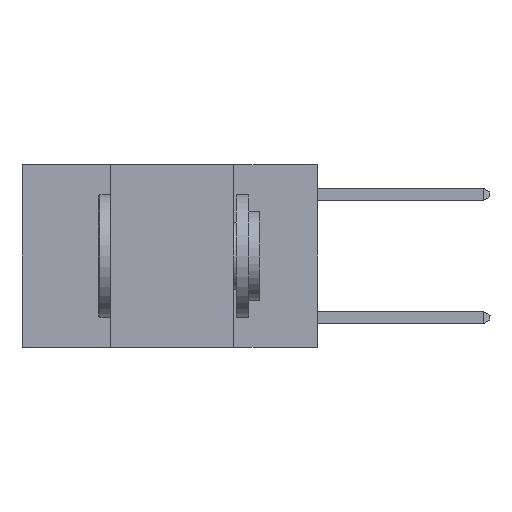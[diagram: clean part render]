
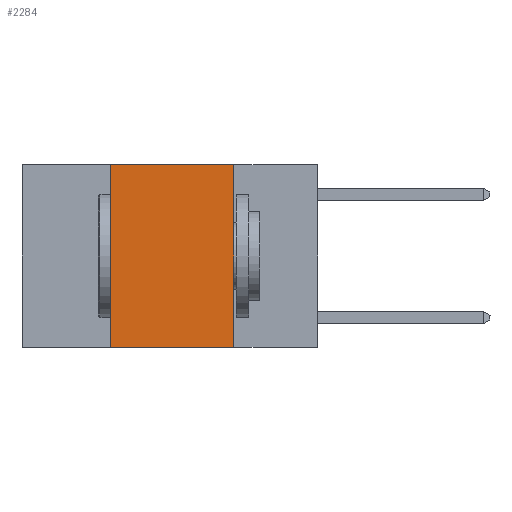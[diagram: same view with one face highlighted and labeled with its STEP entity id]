
A CAD part, left-side view. The second image highlights one B-rep face of the part: STEP entity #2284.
In plain terms, the highlighted planar face has unit normal (-1, 0, 0).
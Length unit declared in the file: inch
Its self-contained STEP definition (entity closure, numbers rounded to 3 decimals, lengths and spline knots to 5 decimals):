
#286 = VERTEX_POINT ( 'NONE', #10735 ) ;
#555 = DIRECTION ( 'NONE',  ( 0., -1., 0. ) ) ;
#801 = CARTESIAN_POINT ( 'NONE',  ( 0., 0.42, 0. ) ) ;
#992 = CARTESIAN_POINT ( 'NONE',  ( 0., 0.17, -0.37 ) ) ;
#1874 = CARTESIAN_POINT ( 'NONE',  ( 0., 0.6, -0.37 ) ) ;
#1924 = VECTOR ( 'NONE', #555, 39.37008 ) ;
#2204 = VERTEX_POINT ( 'NONE', #10578 ) ;
#2284 = ADVANCED_FACE ( 'NONE', ( #10829 ), #9091, .F. ) ;
#3092 = ORIENTED_EDGE ( 'NONE', *, *, #7456, .F. ) ;
#4289 = LINE ( 'NONE', #1874, #8643 ) ;
#4539 = LINE ( 'NONE', #801, #10482 ) ;
#4561 = DIRECTION ( 'NONE',  ( 0., -1., 0. ) ) ;
#4571 = LINE ( 'NONE', #10651, #1924 ) ;
#4818 = CARTESIAN_POINT ( 'NONE',  ( 0., 0.17, 0. ) ) ;
#5016 = AXIS2_PLACEMENT_3D ( 'NONE', #9240, #9254, #7858 ) ;
#6104 = EDGE_CURVE ( 'NONE', #9518, #2204, #4571, .T. ) ;
#6922 = EDGE_CURVE ( 'NONE', #286, #7641, #4289, .T. ) ;
#6931 = DIRECTION ( 'NONE',  ( 0., 0., 1. ) ) ;
#7133 = VECTOR ( 'NONE', #10443, 39.37008 ) ;
#7335 = ORIENTED_EDGE ( 'NONE', *, *, #7977, .F. ) ;
#7456 = EDGE_CURVE ( 'NONE', #286, #9518, #4539, .T. ) ;
#7583 = ORIENTED_EDGE ( 'NONE', *, *, #6922, .T. ) ;
#7641 = VERTEX_POINT ( 'NONE', #992 ) ;
#7858 = DIRECTION ( 'NONE',  ( 0., 0., -1. ) ) ;
#7977 = EDGE_CURVE ( 'NONE', #2204, #7641, #9512, .T. ) ;
#8643 = VECTOR ( 'NONE', #4561, 39.37008 ) ;
#9091 = PLANE ( 'NONE',  #5016 ) ;
#9117 = CARTESIAN_POINT ( 'NONE',  ( 0., 0.42, 0. ) ) ;
#9240 = CARTESIAN_POINT ( 'NONE',  ( 0., 0.6, 0. ) ) ;
#9254 = DIRECTION ( 'NONE',  ( 1., 0., 0. ) ) ;
#9454 = ORIENTED_EDGE ( 'NONE', *, *, #6104, .F. ) ;
#9512 = LINE ( 'NONE', #4818, #7133 ) ;
#9518 = VERTEX_POINT ( 'NONE', #9117 ) ;
#9787 = EDGE_LOOP ( 'NONE', ( #7335, #9454, #3092, #7583 ) ) ;
#10443 = DIRECTION ( 'NONE',  ( 0., 0., -1. ) ) ;
#10482 = VECTOR ( 'NONE', #6931, 39.37008 ) ;
#10578 = CARTESIAN_POINT ( 'NONE',  ( 0., 0.17, 0. ) ) ;
#10651 = CARTESIAN_POINT ( 'NONE',  ( 0., 0.6, 0. ) ) ;
#10735 = CARTESIAN_POINT ( 'NONE',  ( 0., 0.42, -0.37 ) ) ;
#10829 = FACE_OUTER_BOUND ( 'NONE', #9787, .T. ) ;
